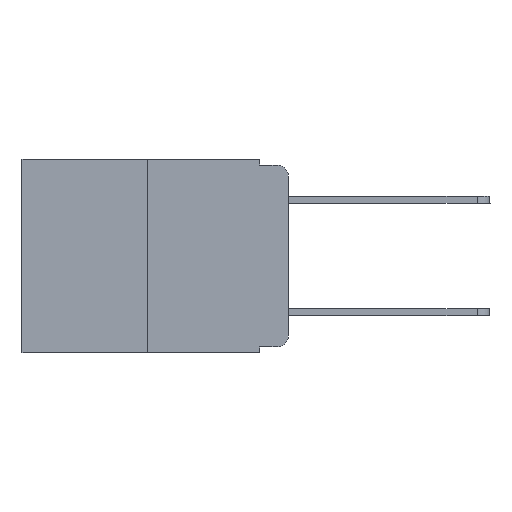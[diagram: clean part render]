
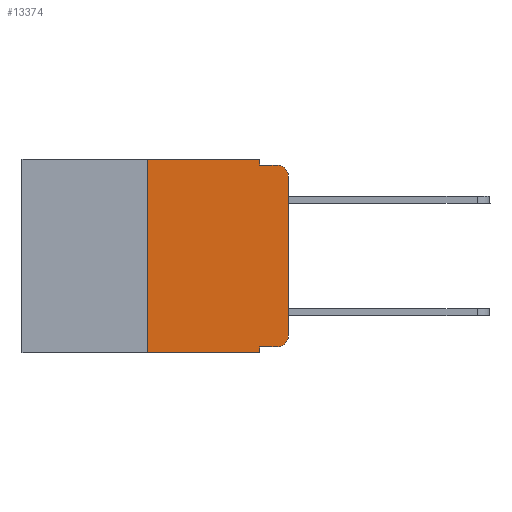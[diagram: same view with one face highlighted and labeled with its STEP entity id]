
A CAD part, left-side view. The second image highlights one B-rep face of the part: STEP entity #13374.
In plain terms, the highlighted planar face has unit normal (-1, 0, 0).
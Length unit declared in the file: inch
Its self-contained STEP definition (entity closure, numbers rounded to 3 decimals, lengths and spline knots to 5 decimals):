
#124 = EDGE_CURVE ( 'NONE', #10354, #20402, #7717, .T. ) ;
#238 = ORIENTED_EDGE ( 'NONE', *, *, #17645, .F. ) ;
#367 = DIRECTION ( 'NONE',  ( 0., -1., 0. ) ) ;
#530 = DIRECTION ( 'NONE',  ( 1., 0., 0. ) ) ;
#748 = VERTEX_POINT ( 'NONE', #9248 ) ;
#1756 = VERTEX_POINT ( 'NONE', #10016 ) ;
#1796 = CARTESIAN_POINT ( 'NONE',  ( 0., 0.051, -0.343 ) ) ;
#2716 = LINE ( 'NONE', #14657, #10060 ) ;
#3251 = EDGE_CURVE ( 'NONE', #10829, #1756, #19858, .T. ) ;
#3487 = DIRECTION ( 'NONE',  ( 0., 0., -1. ) ) ;
#3574 = CARTESIAN_POINT ( 'NONE',  ( 0., 0.473, 0. ) ) ;
#4025 = EDGE_CURVE ( 'NONE', #6475, #23752, #5668, .T. ) ;
#4135 = CARTESIAN_POINT ( 'NONE',  ( 0., 0.473, 0. ) ) ;
#4645 = EDGE_CURVE ( 'NONE', #14909, #22890, #2716, .T. ) ;
#4759 = EDGE_CURVE ( 'NONE', #23752, #9669, #11512, .T. ) ;
#4783 = LINE ( 'NONE', #24065, #22994 ) ;
#5101 = CARTESIAN_POINT ( 'NONE',  ( 0., 0.02, -0.03 ) ) ;
#5196 = EDGE_LOOP ( 'NONE', ( #6957, #11356, #5366, #238, #14924, #19414, #15910, #8243, #12859, #17207 ) ) ;
#5366 = ORIENTED_EDGE ( 'NONE', *, *, #3251, .F. ) ;
#5668 = LINE ( 'NONE', #8685, #23296 ) ;
#5951 = LINE ( 'NONE', #16100, #15361 ) ;
#6475 = VERTEX_POINT ( 'NONE', #8456 ) ;
#6493 = DIRECTION ( 'NONE',  ( 0., 0., 1. ) ) ;
#6878 = CARTESIAN_POINT ( 'NONE',  ( 0., 0.051, -0.333 ) ) ;
#6957 = ORIENTED_EDGE ( 'NONE', *, *, #20500, .T. ) ;
#7163 = CARTESIAN_POINT ( 'NONE',  ( 0., 0.051, 0. ) ) ;
#7295 = DIRECTION ( 'NONE',  ( 0., -1., 0. ) ) ;
#7705 = DIRECTION ( 'NONE',  ( 0., 0., 1. ) ) ;
#7717 = CIRCLE ( 'NONE', #8641, 0.02 ) ;
#8243 = ORIENTED_EDGE ( 'NONE', *, *, #4645, .F. ) ;
#8456 = CARTESIAN_POINT ( 'NONE',  ( 0., 0.25, -0.343 ) ) ;
#8641 = AXIS2_PLACEMENT_3D ( 'NONE', #15731, #10435, #17856 ) ;
#8644 = VECTOR ( 'NONE', #21084, 39.37008 ) ;
#8685 = CARTESIAN_POINT ( 'NONE',  ( 0., 0.25, 0. ) ) ;
#8717 = VECTOR ( 'NONE', #7705, 39.37008 ) ;
#8756 = DIRECTION ( 'NONE',  ( 0., -1., 0. ) ) ;
#9248 = CARTESIAN_POINT ( 'NONE',  ( 0., 0., -0.03 ) ) ;
#9669 = VERTEX_POINT ( 'NONE', #17027 ) ;
#9797 = DIRECTION ( 'NONE',  ( 0., 0., -1. ) ) ;
#9943 = FACE_OUTER_BOUND ( 'NONE', #5196, .T. ) ;
#10016 = CARTESIAN_POINT ( 'NONE',  ( 0., 0.02, -0.01 ) ) ;
#10060 = VECTOR ( 'NONE', #3487, 39.37008 ) ;
#10354 = VERTEX_POINT ( 'NONE', #13685 ) ;
#10435 = DIRECTION ( 'NONE',  ( -1., 0., 0. ) ) ;
#10829 = VERTEX_POINT ( 'NONE', #12165 ) ;
#11062 = EDGE_CURVE ( 'NONE', #6475, #22890, #4783, .T. ) ;
#11356 = ORIENTED_EDGE ( 'NONE', *, *, #19756, .T. ) ;
#11428 = PLANE ( 'NONE',  #15360 ) ;
#11512 = LINE ( 'NONE', #3574, #16808 ) ;
#12165 = CARTESIAN_POINT ( 'NONE',  ( 0., 0.051, -0.01 ) ) ;
#12707 = AXIS2_PLACEMENT_3D ( 'NONE', #5101, #14449, #14619 ) ;
#12859 = ORIENTED_EDGE ( 'NONE', *, *, #23984, .T. ) ;
#12879 = CARTESIAN_POINT ( 'NONE',  ( 0., 0., -0.313 ) ) ;
#13374 = ADVANCED_FACE ( 'NONE', ( #9943 ), #11428, .F. ) ;
#13685 = CARTESIAN_POINT ( 'NONE',  ( 0., 0.02, -0.333 ) ) ;
#14449 = DIRECTION ( 'NONE',  ( -1., 0., 0. ) ) ;
#14594 = LINE ( 'NONE', #19172, #8717 ) ;
#14619 = DIRECTION ( 'NONE',  ( 0., 0., -1. ) ) ;
#14643 = CIRCLE ( 'NONE', #12707, 0.02 ) ;
#14657 = CARTESIAN_POINT ( 'NONE',  ( 0., 0.051, 0. ) ) ;
#14909 = VERTEX_POINT ( 'NONE', #6878 ) ;
#14924 = ORIENTED_EDGE ( 'NONE', *, *, #4759, .F. ) ;
#15360 = AXIS2_PLACEMENT_3D ( 'NONE', #4135, #530, #9797 ) ;
#15361 = VECTOR ( 'NONE', #8756, 39.37008 ) ;
#15731 = CARTESIAN_POINT ( 'NONE',  ( 0., 0.02, -0.313 ) ) ;
#15910 = ORIENTED_EDGE ( 'NONE', *, *, #11062, .T. ) ;
#15917 = VECTOR ( 'NONE', #20593, 39.37008 ) ;
#16100 = CARTESIAN_POINT ( 'NONE',  ( 0., 0.051, -0.333 ) ) ;
#16208 = LINE ( 'NONE', #7163, #15917 ) ;
#16808 = VECTOR ( 'NONE', #367, 39.37008 ) ;
#17027 = CARTESIAN_POINT ( 'NONE',  ( 0., 0.051, 0. ) ) ;
#17207 = ORIENTED_EDGE ( 'NONE', *, *, #124, .T. ) ;
#17645 = EDGE_CURVE ( 'NONE', #9669, #10829, #16208, .T. ) ;
#17856 = DIRECTION ( 'NONE',  ( 0., 0., -1. ) ) ;
#19172 = CARTESIAN_POINT ( 'NONE',  ( 0., 0., 0. ) ) ;
#19289 = CARTESIAN_POINT ( 'NONE',  ( 0., 0.051, -0.01 ) ) ;
#19414 = ORIENTED_EDGE ( 'NONE', *, *, #4025, .F. ) ;
#19756 = EDGE_CURVE ( 'NONE', #748, #1756, #14643, .T. ) ;
#19858 = LINE ( 'NONE', #19289, #8644 ) ;
#20402 = VERTEX_POINT ( 'NONE', #12879 ) ;
#20500 = EDGE_CURVE ( 'NONE', #20402, #748, #14594, .T. ) ;
#20593 = DIRECTION ( 'NONE',  ( 0., 0., -1. ) ) ;
#20979 = CARTESIAN_POINT ( 'NONE',  ( 0., 0.25, 0. ) ) ;
#21084 = DIRECTION ( 'NONE',  ( 0., -1., 0. ) ) ;
#22890 = VERTEX_POINT ( 'NONE', #1796 ) ;
#22994 = VECTOR ( 'NONE', #7295, 39.37008 ) ;
#23296 = VECTOR ( 'NONE', #6493, 39.37008 ) ;
#23752 = VERTEX_POINT ( 'NONE', #20979 ) ;
#23984 = EDGE_CURVE ( 'NONE', #14909, #10354, #5951, .T. ) ;
#24065 = CARTESIAN_POINT ( 'NONE',  ( 0., 0.473, -0.343 ) ) ;
